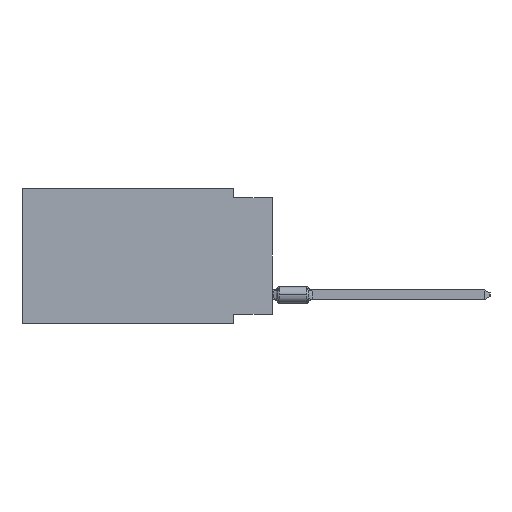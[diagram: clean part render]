
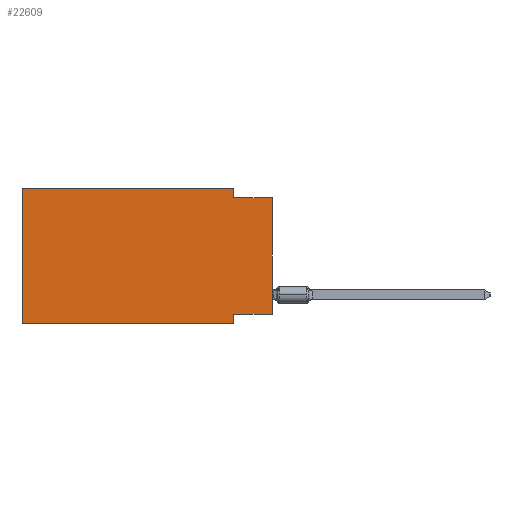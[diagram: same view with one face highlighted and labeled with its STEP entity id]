
A CAD part, left-side view. The second image highlights one B-rep face of the part: STEP entity #22609.
In plain terms, the highlighted planar face has unit normal (-1, 0, 0).
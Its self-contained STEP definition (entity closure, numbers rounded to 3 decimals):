
#40 = CARTESIAN_POINT ( 'NONE',  ( 0., 2.54, -8.255 ) ) ;
#1771 = DIRECTION ( 'NONE',  ( 0., -1., 0. ) ) ;
#1809 = LINE ( 'NONE', #25092, #12402 ) ;
#2338 = PLANE ( 'NONE',  #17259 ) ;
#2495 = LINE ( 'NONE', #17329, #3722 ) ;
#3479 = LINE ( 'NONE', #24549, #3550 ) ;
#3550 = VECTOR ( 'NONE', #9317, 1000. ) ;
#3722 = VECTOR ( 'NONE', #13178, 1000. ) ;
#3898 = DIRECTION ( 'NONE',  ( 0., 1., 0. ) ) ;
#3987 = VECTOR ( 'NONE', #1771, 1000. ) ;
#4492 = ORIENTED_EDGE ( 'NONE', *, *, #5631, .T. ) ;
#4907 = ORIENTED_EDGE ( 'NONE', *, *, #21049, .F. ) ;
#4935 = ORIENTED_EDGE ( 'NONE', *, *, #5806, .F. ) ;
#5631 = EDGE_CURVE ( 'NONE', #22276, #26647, #23407, .T. ) ;
#5659 = EDGE_CURVE ( 'NONE', #25916, #5988, #16647, .T. ) ;
#5806 = EDGE_CURVE ( 'NONE', #12043, #5988, #2495, .T. ) ;
#5988 = VERTEX_POINT ( 'NONE', #24765 ) ;
#6079 = DIRECTION ( 'NONE',  ( 0., 0., -1. ) ) ;
#6196 = CARTESIAN_POINT ( 'NONE',  ( 0., 16.383, 0. ) ) ;
#8068 = CARTESIAN_POINT ( 'NONE',  ( 0., 0., -8.255 ) ) ;
#8442 = DIRECTION ( 'NONE',  ( 0., -1., 0. ) ) ;
#8864 = ORIENTED_EDGE ( 'NONE', *, *, #23645, .F. ) ;
#9317 = DIRECTION ( 'NONE',  ( 0., 0., -1. ) ) ;
#9689 = EDGE_CURVE ( 'NONE', #25916, #20682, #14585, .T. ) ;
#10404 = CARTESIAN_POINT ( 'NONE',  ( 0., 0., 0. ) ) ;
#10845 = EDGE_CURVE ( 'NONE', #22276, #12892, #14279, .T. ) ;
#11912 = CARTESIAN_POINT ( 'NONE',  ( 0., 16.383, 0. ) ) ;
#12043 = VERTEX_POINT ( 'NONE', #25983 ) ;
#12402 = VECTOR ( 'NONE', #21090, 1000. ) ;
#12475 = CARTESIAN_POINT ( 'NONE',  ( 0., 16.383, -8.89 ) ) ;
#12752 = ORIENTED_EDGE ( 'NONE', *, *, #10845, .F. ) ;
#12888 = DIRECTION ( 'NONE',  ( 0., 0., 1. ) ) ;
#12892 = VERTEX_POINT ( 'NONE', #22604 ) ;
#13178 = DIRECTION ( 'NONE',  ( 0., -1., 0. ) ) ;
#14279 = LINE ( 'NONE', #11912, #16261 ) ;
#14585 = LINE ( 'NONE', #8068, #26812 ) ;
#14960 = FACE_OUTER_BOUND ( 'NONE', #26508, .T. ) ;
#15084 = CARTESIAN_POINT ( 'NONE',  ( 0., 16.383, 0. ) ) ;
#16261 = VECTOR ( 'NONE', #18294, 1000. ) ;
#16427 = CARTESIAN_POINT ( 'NONE',  ( 0., 16.383, -8.89 ) ) ;
#16479 = ORIENTED_EDGE ( 'NONE', *, *, #9689, .F. ) ;
#16647 = LINE ( 'NONE', #10404, #18035 ) ;
#17259 = AXIS2_PLACEMENT_3D ( 'NONE', #15084, #23387, #6079 ) ;
#17329 = CARTESIAN_POINT ( 'NONE',  ( 0., 0., -0.635 ) ) ;
#17614 = CARTESIAN_POINT ( 'NONE',  ( 0., 0., -8.255 ) ) ;
#18035 = VECTOR ( 'NONE', #12888, 1000. ) ;
#18294 = DIRECTION ( 'NONE',  ( 0., 0., 1. ) ) ;
#20682 = VERTEX_POINT ( 'NONE', #40 ) ;
#21049 = EDGE_CURVE ( 'NONE', #26897, #12043, #1809, .T. ) ;
#21090 = DIRECTION ( 'NONE',  ( 0., 0., -1. ) ) ;
#22276 = VERTEX_POINT ( 'NONE', #16427 ) ;
#22604 = CARTESIAN_POINT ( 'NONE',  ( 0., 16.383, 0. ) ) ;
#22609 = ADVANCED_FACE ( 'NONE', ( #14960 ), #2338, .F. ) ;
#22718 = ORIENTED_EDGE ( 'NONE', *, *, #5659, .T. ) ;
#23101 = LINE ( 'NONE', #6196, #3987 ) ;
#23294 = CARTESIAN_POINT ( 'NONE',  ( 0., 2.54, 0. ) ) ;
#23332 = VECTOR ( 'NONE', #8442, 1000. ) ;
#23387 = DIRECTION ( 'NONE',  ( 1., 0., 0. ) ) ;
#23407 = LINE ( 'NONE', #12475, #23332 ) ;
#23485 = CARTESIAN_POINT ( 'NONE',  ( 0., 2.54, -8.89 ) ) ;
#23645 = EDGE_CURVE ( 'NONE', #20682, #26647, #3479, .T. ) ;
#24046 = EDGE_CURVE ( 'NONE', #12892, #26897, #23101, .T. ) ;
#24549 = CARTESIAN_POINT ( 'NONE',  ( 0., 2.54, -8.89 ) ) ;
#24765 = CARTESIAN_POINT ( 'NONE',  ( 0., 0., -0.635 ) ) ;
#25092 = CARTESIAN_POINT ( 'NONE',  ( 0., 2.54, 0. ) ) ;
#25916 = VERTEX_POINT ( 'NONE', #17614 ) ;
#25983 = CARTESIAN_POINT ( 'NONE',  ( 0., 2.54, -0.635 ) ) ;
#26370 = ORIENTED_EDGE ( 'NONE', *, *, #24046, .F. ) ;
#26508 = EDGE_LOOP ( 'NONE', ( #22718, #4935, #4907, #26370, #12752, #4492, #8864, #16479 ) ) ;
#26647 = VERTEX_POINT ( 'NONE', #23485 ) ;
#26812 = VECTOR ( 'NONE', #3898, 1000. ) ;
#26897 = VERTEX_POINT ( 'NONE', #23294 ) ;
